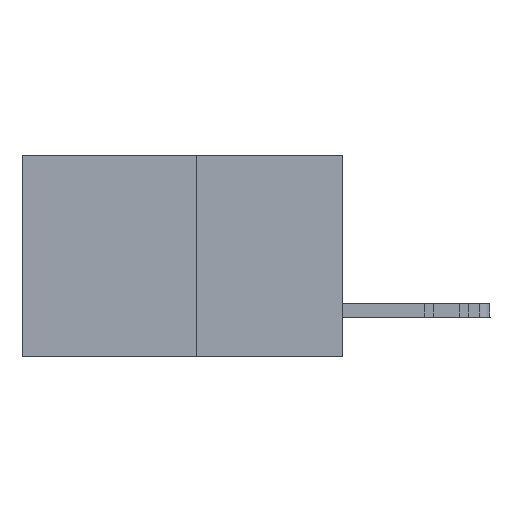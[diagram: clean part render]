
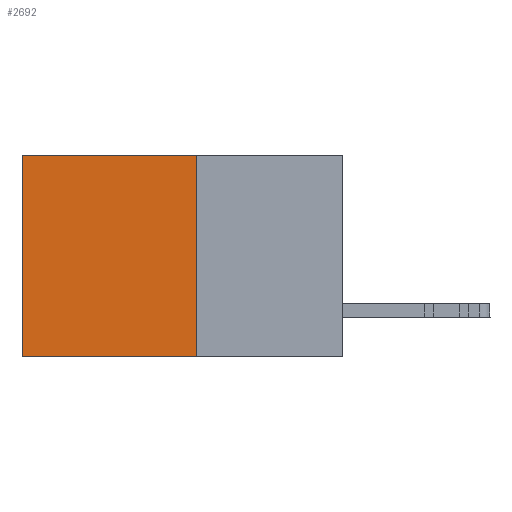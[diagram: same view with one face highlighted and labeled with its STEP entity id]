
A CAD part, left-side view. The second image highlights one B-rep face of the part: STEP entity #2692.
In plain terms, the highlighted planar face has unit normal (-1, 0, 0).
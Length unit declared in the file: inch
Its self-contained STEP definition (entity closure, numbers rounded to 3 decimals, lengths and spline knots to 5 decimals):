
#583 = VECTOR ( 'NONE', #22375, 39.37008 ) ;
#1043 = VECTOR ( 'NONE', #32674, 39.37008 ) ;
#1211 = VERTEX_POINT ( 'NONE', #9376 ) ;
#2692 = ADVANCED_FACE ( 'NONE', ( #22362 ), #18724, .F. ) ;
#2913 = CARTESIAN_POINT ( 'NONE',  ( 0.277, 0.59, -0.37 ) ) ;
#4173 = CARTESIAN_POINT ( 'NONE',  ( 0.277, 0.59, -0.37 ) ) ;
#5693 = DIRECTION ( 'NONE',  ( 0., 0., -1. ) ) ;
#8350 = LINE ( 'NONE', #2913, #14389 ) ;
#9376 = CARTESIAN_POINT ( 'NONE',  ( 0.277, 0.27, -0.37 ) ) ;
#9780 = DIRECTION ( 'NONE',  ( 1., 0., 0. ) ) ;
#10518 = EDGE_CURVE ( 'NONE', #1211, #19701, #26303, .T. ) ;
#11638 = ORIENTED_EDGE ( 'NONE', *, *, #10518, .F. ) ;
#11974 = ORIENTED_EDGE ( 'NONE', *, *, #23018, .F. ) ;
#14026 = LINE ( 'NONE', #14824, #1043 ) ;
#14062 = VERTEX_POINT ( 'NONE', #16949 ) ;
#14389 = VECTOR ( 'NONE', #23512, 39.37008 ) ;
#14824 = CARTESIAN_POINT ( 'NONE',  ( 0.277, 0.27, 0. ) ) ;
#14869 = VERTEX_POINT ( 'NONE', #30508 ) ;
#14897 = AXIS2_PLACEMENT_3D ( 'NONE', #17914, #9780, #5693 ) ;
#16273 = DIRECTION ( 'NONE',  ( 0., 1., 0. ) ) ;
#16949 = CARTESIAN_POINT ( 'NONE',  ( 0.277, 0.59, 0. ) ) ;
#17914 = CARTESIAN_POINT ( 'NONE',  ( 0.277, 0.27, -0.37 ) ) ;
#18724 = PLANE ( 'NONE',  #14897 ) ;
#19398 = EDGE_LOOP ( 'NONE', ( #32165, #11638, #11974, #30375 ) ) ;
#19476 = VECTOR ( 'NONE', #16273, 39.37008 ) ;
#19701 = VERTEX_POINT ( 'NONE', #4173 ) ;
#19772 = CARTESIAN_POINT ( 'NONE',  ( 0.277, 0.27, -0.37 ) ) ;
#21149 = LINE ( 'NONE', #19772, #583 ) ;
#22335 = EDGE_CURVE ( 'NONE', #14869, #14062, #14026, .T. ) ;
#22362 = FACE_OUTER_BOUND ( 'NONE', #19398, .T. ) ;
#22375 = DIRECTION ( 'NONE',  ( 0., 0., -1. ) ) ;
#23018 = EDGE_CURVE ( 'NONE', #14869, #1211, #21149, .T. ) ;
#23512 = DIRECTION ( 'NONE',  ( 0., 0., -1. ) ) ;
#26303 = LINE ( 'NONE', #28977, #19476 ) ;
#28977 = CARTESIAN_POINT ( 'NONE',  ( 0.277, 0.27, -0.37 ) ) ;
#30375 = ORIENTED_EDGE ( 'NONE', *, *, #22335, .T. ) ;
#30508 = CARTESIAN_POINT ( 'NONE',  ( 0.277, 0.27, 0. ) ) ;
#32165 = ORIENTED_EDGE ( 'NONE', *, *, #32321, .T. ) ;
#32321 = EDGE_CURVE ( 'NONE', #14062, #19701, #8350, .T. ) ;
#32674 = DIRECTION ( 'NONE',  ( 0., 1., 0. ) ) ;
